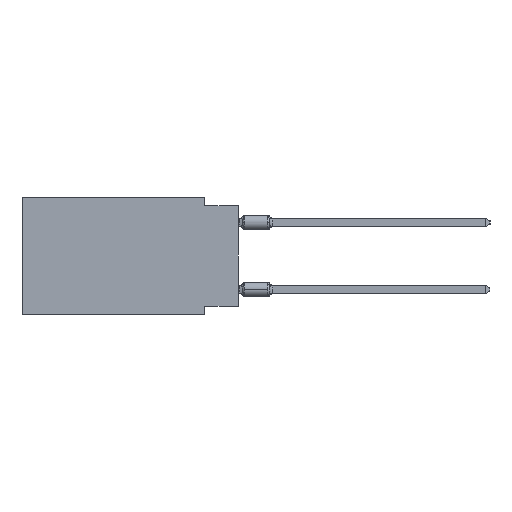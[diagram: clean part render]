
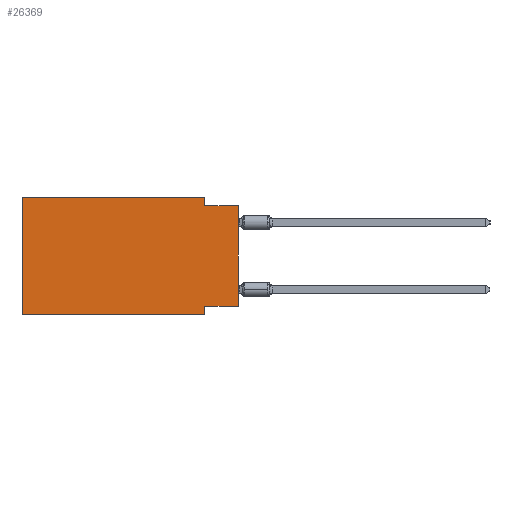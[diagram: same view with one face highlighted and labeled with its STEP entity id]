
A CAD part, left-side view. The second image highlights one B-rep face of the part: STEP entity #26369.
In plain terms, the highlighted planar face has unit normal (-1, 0, 0).
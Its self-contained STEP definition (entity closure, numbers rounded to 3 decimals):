
#109 = VECTOR ( 'NONE', #2930, 1000. ) ;
#1000 = CARTESIAN_POINT ( 'NONE',  ( 0., 16.383, 0. ) ) ;
#1697 = CARTESIAN_POINT ( 'NONE',  ( 0., 2.54, -8.89 ) ) ;
#2000 = VECTOR ( 'NONE', #21492, 1000. ) ;
#2719 = VERTEX_POINT ( 'NONE', #18913 ) ;
#2930 = DIRECTION ( 'NONE',  ( 0., 0., 1. ) ) ;
#3039 = VERTEX_POINT ( 'NONE', #9440 ) ;
#3815 = ORIENTED_EDGE ( 'NONE', *, *, #9287, .F. ) ;
#5190 = CARTESIAN_POINT ( 'NONE',  ( 0., 0., 0. ) ) ;
#5964 = ORIENTED_EDGE ( 'NONE', *, *, #28961, .T. ) ;
#6273 = DIRECTION ( 'NONE',  ( 1., 0., 0. ) ) ;
#6306 = ORIENTED_EDGE ( 'NONE', *, *, #25326, .F. ) ;
#7004 = PLANE ( 'NONE',  #33849 ) ;
#7562 = DIRECTION ( 'NONE',  ( 0., -1., 0. ) ) ;
#8127 = DIRECTION ( 'NONE',  ( 0., -1., 0. ) ) ;
#9022 = VERTEX_POINT ( 'NONE', #9727 ) ;
#9287 = EDGE_CURVE ( 'NONE', #18383, #26800, #13775, .T. ) ;
#9440 = CARTESIAN_POINT ( 'NONE',  ( 0., 16.383, 0. ) ) ;
#9727 = CARTESIAN_POINT ( 'NONE',  ( 0., 0., -0.635 ) ) ;
#10649 = CARTESIAN_POINT ( 'NONE',  ( 0., 0., -8.255 ) ) ;
#11683 = CARTESIAN_POINT ( 'NONE',  ( 0., 2.54, 0. ) ) ;
#11833 = CARTESIAN_POINT ( 'NONE',  ( 0., 16.383, 0. ) ) ;
#12065 = VECTOR ( 'NONE', #36599, 1000. ) ;
#13006 = LINE ( 'NONE', #1697, #31101 ) ;
#13775 = LINE ( 'NONE', #25254, #12065 ) ;
#14537 = CARTESIAN_POINT ( 'NONE',  ( 0., 16.383, -8.89 ) ) ;
#14717 = LINE ( 'NONE', #1000, #34864 ) ;
#17015 = LINE ( 'NONE', #30584, #109 ) ;
#17242 = LINE ( 'NONE', #11683, #2000 ) ;
#17762 = VECTOR ( 'NONE', #7562, 1000. ) ;
#18035 = ORIENTED_EDGE ( 'NONE', *, *, #18061, .F. ) ;
#18061 = EDGE_CURVE ( 'NONE', #23232, #3039, #17015, .T. ) ;
#18109 = EDGE_CURVE ( 'NONE', #2719, #9022, #22044, .T. ) ;
#18383 = VERTEX_POINT ( 'NONE', #10649 ) ;
#18864 = CARTESIAN_POINT ( 'NONE',  ( 0., 16.383, -8.89 ) ) ;
#18913 = CARTESIAN_POINT ( 'NONE',  ( 0., 2.54, -0.635 ) ) ;
#19987 = CARTESIAN_POINT ( 'NONE',  ( 0., 2.54, 0. ) ) ;
#20540 = DIRECTION ( 'NONE',  ( 0., 0., -1. ) ) ;
#21492 = DIRECTION ( 'NONE',  ( 0., 0., -1. ) ) ;
#21934 = EDGE_CURVE ( 'NONE', #3039, #34836, #14717, .T. ) ;
#22032 = CARTESIAN_POINT ( 'NONE',  ( 0., 2.54, -8.89 ) ) ;
#22044 = LINE ( 'NONE', #33377, #26166 ) ;
#23232 = VERTEX_POINT ( 'NONE', #14537 ) ;
#23256 = DIRECTION ( 'NONE',  ( 0., -1., 0. ) ) ;
#24373 = VERTEX_POINT ( 'NONE', #22032 ) ;
#24406 = VECTOR ( 'NONE', #25889, 1000. ) ;
#24445 = LINE ( 'NONE', #18864, #17762 ) ;
#25254 = CARTESIAN_POINT ( 'NONE',  ( 0., 0., -8.255 ) ) ;
#25326 = EDGE_CURVE ( 'NONE', #34836, #2719, #17242, .T. ) ;
#25889 = DIRECTION ( 'NONE',  ( 0., 0., 1. ) ) ;
#26166 = VECTOR ( 'NONE', #8127, 1000. ) ;
#26369 = ADVANCED_FACE ( 'NONE', ( #32423 ), #7004, .F. ) ;
#26625 = CARTESIAN_POINT ( 'NONE',  ( 0., 2.54, -8.255 ) ) ;
#26800 = VERTEX_POINT ( 'NONE', #26625 ) ;
#26869 = ORIENTED_EDGE ( 'NONE', *, *, #18109, .F. ) ;
#26938 = DIRECTION ( 'NONE',  ( 0., 0., -1. ) ) ;
#28961 = EDGE_CURVE ( 'NONE', #18383, #9022, #31660, .T. ) ;
#29716 = ORIENTED_EDGE ( 'NONE', *, *, #21934, .F. ) ;
#29808 = ORIENTED_EDGE ( 'NONE', *, *, #31706, .F. ) ;
#30584 = CARTESIAN_POINT ( 'NONE',  ( 0., 16.383, 0. ) ) ;
#31101 = VECTOR ( 'NONE', #26938, 1000. ) ;
#31170 = ORIENTED_EDGE ( 'NONE', *, *, #36390, .T. ) ;
#31660 = LINE ( 'NONE', #5190, #24406 ) ;
#31706 = EDGE_CURVE ( 'NONE', #26800, #24373, #13006, .T. ) ;
#32423 = FACE_OUTER_BOUND ( 'NONE', #34469, .T. ) ;
#33377 = CARTESIAN_POINT ( 'NONE',  ( 0., 0., -0.635 ) ) ;
#33849 = AXIS2_PLACEMENT_3D ( 'NONE', #11833, #6273, #20540 ) ;
#34469 = EDGE_LOOP ( 'NONE', ( #5964, #26869, #6306, #29716, #18035, #31170, #29808, #3815 ) ) ;
#34836 = VERTEX_POINT ( 'NONE', #19987 ) ;
#34864 = VECTOR ( 'NONE', #23256, 1000. ) ;
#36390 = EDGE_CURVE ( 'NONE', #23232, #24373, #24445, .T. ) ;
#36599 = DIRECTION ( 'NONE',  ( 0., 1., 0. ) ) ;
